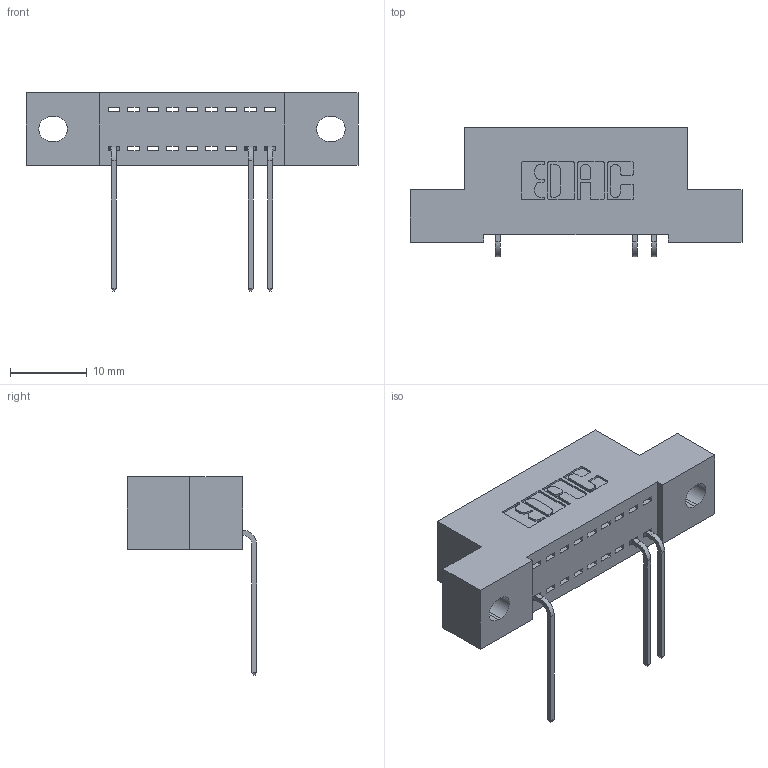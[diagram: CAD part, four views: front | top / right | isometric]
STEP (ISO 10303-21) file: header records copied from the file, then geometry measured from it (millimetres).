
FILE_DESCRIPTION (( 'STEP AP203' ), '1' );
FILE_NAME ('392-009-559-102.STEP', '2018-08-14T19:59:58', ( '' ), ( '' ), 'SwSTEP 2.0', 'SolidWorks 2016', '' );
FILE_SCHEMA (( 'CONFIG_CONTROL_DESIGN' ));
Length unit declared in the file: inch
Products named in the file (3): 342 Part_.128 Slot; 345-292-001_558 559 Tail - 1; 392-009-559-102
Assembly tree (4 placements, depth 2):
  392-009-559-102
    342 Part_.128 Slot
    345-292-001_558 559 Tail - 1  x3
Bounding box: 43.18 x 16.83 x 25.78 mm (x, y, z)
Volume: 3553.7 mm3; surface area: 4063.1 mm2
Topology: 4 solids, 4 shells, 366 faces, 1109 edges, 734 vertices
Faces by surface type: plane 274, cylinder 92
Entity records: 9665 total; most frequent: CARTESIAN_POINT 1707, ORIENTED_EDGE 1658, DIRECTION 1499, EDGE_CURVE 829, LINE 701, VECTOR 701, VERTEX_POINT 550, AXIS2_PLACEMENT_3D 399
